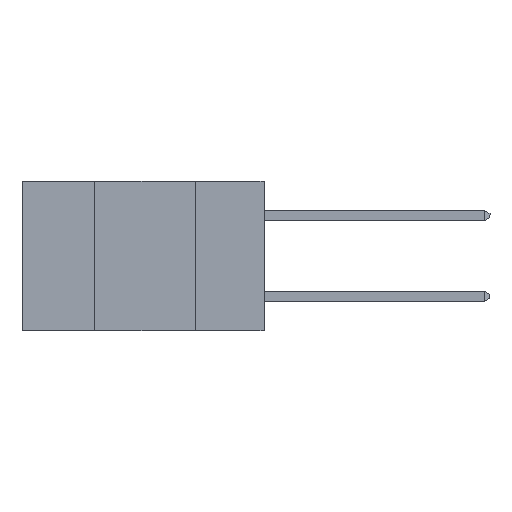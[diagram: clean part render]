
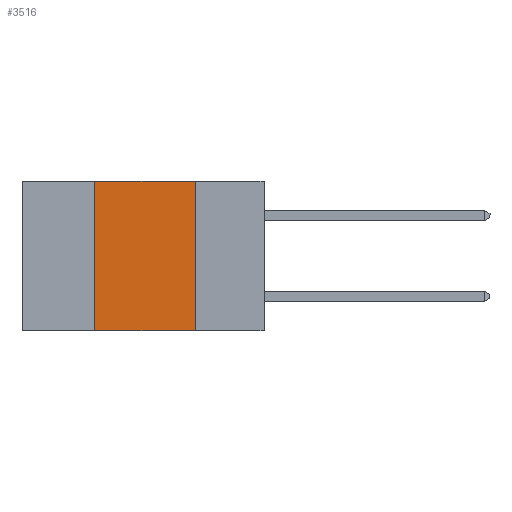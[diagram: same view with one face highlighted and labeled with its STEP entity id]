
A CAD part, left-side view. The second image highlights one B-rep face of the part: STEP entity #3516.
In plain terms, the highlighted planar face has unit normal (-1, 0, 0).
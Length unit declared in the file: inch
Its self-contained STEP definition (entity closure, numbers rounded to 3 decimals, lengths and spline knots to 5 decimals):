
#743 = VECTOR ( 'NONE', #1668, 39.37008 ) ;
#758 = CARTESIAN_POINT ( 'NONE',  ( 0., 0.6, 0. ) ) ;
#1397 = LINE ( 'NONE', #3722, #743 ) ;
#1668 = DIRECTION ( 'NONE',  ( 0., 0., 1. ) ) ;
#3516 = ADVANCED_FACE ( 'NONE', ( #5720 ), #22764, .F. ) ;
#3722 = CARTESIAN_POINT ( 'NONE',  ( 0., 0.42, 0. ) ) ;
#3845 = CARTESIAN_POINT ( 'NONE',  ( 0., 0.42, -0.37 ) ) ;
#4601 = VECTOR ( 'NONE', #15832, 39.37008 ) ;
#4617 = ORIENTED_EDGE ( 'NONE', *, *, #20136, .F. ) ;
#4648 = ORIENTED_EDGE ( 'NONE', *, *, #13612, .F. ) ;
#5059 = CARTESIAN_POINT ( 'NONE',  ( 0., 0.6, 0. ) ) ;
#5720 = FACE_OUTER_BOUND ( 'NONE', #20903, .T. ) ;
#7834 = LINE ( 'NONE', #12212, #25056 ) ;
#8094 = CARTESIAN_POINT ( 'NONE',  ( 0., 0.17, -0.37 ) ) ;
#8145 = VERTEX_POINT ( 'NONE', #17575 ) ;
#8180 = VERTEX_POINT ( 'NONE', #3845 ) ;
#8773 = DIRECTION ( 'NONE',  ( 1., 0., 0. ) ) ;
#10039 = EDGE_CURVE ( 'NONE', #10851, #8145, #10389, .T. ) ;
#10172 = ORIENTED_EDGE ( 'NONE', *, *, #10039, .F. ) ;
#10389 = LINE ( 'NONE', #758, #26268 ) ;
#10851 = VERTEX_POINT ( 'NONE', #18329 ) ;
#11453 = LINE ( 'NONE', #13694, #4601 ) ;
#12212 = CARTESIAN_POINT ( 'NONE',  ( 0., 0.6, -0.37 ) ) ;
#13612 = EDGE_CURVE ( 'NONE', #8180, #10851, #1397, .T. ) ;
#13694 = CARTESIAN_POINT ( 'NONE',  ( 0., 0.17, 0. ) ) ;
#15425 = VERTEX_POINT ( 'NONE', #8094 ) ;
#15832 = DIRECTION ( 'NONE',  ( 0., 0., -1. ) ) ;
#16081 = ORIENTED_EDGE ( 'NONE', *, *, #26601, .T. ) ;
#16810 = DIRECTION ( 'NONE',  ( 0., 0., -1. ) ) ;
#17575 = CARTESIAN_POINT ( 'NONE',  ( 0., 0.17, 0. ) ) ;
#18329 = CARTESIAN_POINT ( 'NONE',  ( 0., 0.42, 0. ) ) ;
#20136 = EDGE_CURVE ( 'NONE', #8145, #15425, #11453, .T. ) ;
#20903 = EDGE_LOOP ( 'NONE', ( #4617, #10172, #4648, #16081 ) ) ;
#22764 = PLANE ( 'NONE',  #24837 ) ;
#24837 = AXIS2_PLACEMENT_3D ( 'NONE', #5059, #8773, #16810 ) ;
#25056 = VECTOR ( 'NONE', #26679, 39.37008 ) ;
#25774 = DIRECTION ( 'NONE',  ( 0., -1., 0. ) ) ;
#26268 = VECTOR ( 'NONE', #25774, 39.37008 ) ;
#26601 = EDGE_CURVE ( 'NONE', #8180, #15425, #7834, .T. ) ;
#26679 = DIRECTION ( 'NONE',  ( 0., -1., 0. ) ) ;
